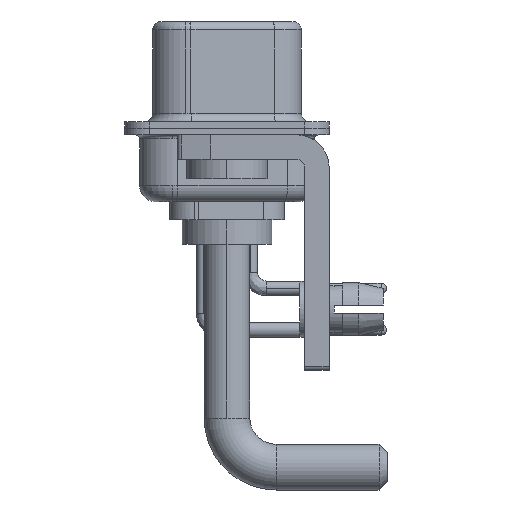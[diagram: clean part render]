
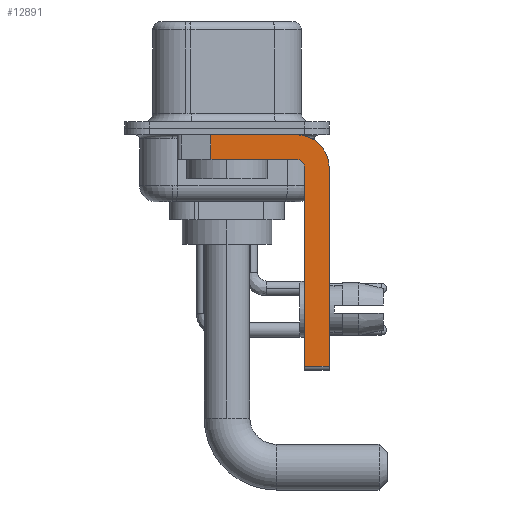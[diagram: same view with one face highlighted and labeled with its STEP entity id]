
A CAD part, left-side view. The second image highlights one B-rep face of the part: STEP entity #12891.
In plain terms, the highlighted planar face has unit normal (-1, 0, 0).
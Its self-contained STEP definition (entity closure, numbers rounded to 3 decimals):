
#320 = CARTESIAN_POINT ( 'NONE',  ( -2.9, -4.25, -2.4 ) ) ;
#941 = ORIENTED_EDGE ( 'NONE', *, *, #22098, .T. ) ;
#2034 = VECTOR ( 'NONE', #27669, 1000. ) ;
#2290 = CARTESIAN_POINT ( 'NONE',  ( -2.9, -4.25, -14.55 ) ) ;
#2913 = LINE ( 'NONE', #7847, #25503 ) ;
#4071 = CARTESIAN_POINT ( 'NONE',  ( -2.9, 0.978, -1.9 ) ) ;
#4389 = ORIENTED_EDGE ( 'NONE', *, *, #28642, .F. ) ;
#4575 = CARTESIAN_POINT ( 'NONE',  ( -2.9, -4.25, -2.4 ) ) ;
#4962 = PLANE ( 'NONE',  #6424 ) ;
#5772 = CARTESIAN_POINT ( 'NONE',  ( -2.9, -4.25, -1.9 ) ) ;
#6424 = AXIS2_PLACEMENT_3D ( 'NONE', #320, #7862, #24364 ) ;
#6675 = EDGE_CURVE ( 'NONE', #24162, #13296, #2913, .T. ) ;
#6744 = VECTOR ( 'NONE', #20681, 1000. ) ;
#7289 = VERTEX_POINT ( 'NONE', #16029 ) ;
#7725 = EDGE_CURVE ( 'NONE', #24919, #7289, #20651, .T. ) ;
#7847 = CARTESIAN_POINT ( 'NONE',  ( -2.9, 0.978, -1.9 ) ) ;
#7862 = DIRECTION ( 'NONE',  ( 1., 0., 0. ) ) ;
#8872 = CARTESIAN_POINT ( 'NONE',  ( -2.9, -4.25, -1.9 ) ) ;
#8944 = CARTESIAN_POINT ( 'NONE',  ( -2.9, -4.75, -14.8 ) ) ;
#10018 = EDGE_LOOP ( 'NONE', ( #18053, #20762, #11144, #4389, #27087, #941, #21379, #15560 ) ) ;
#11144 = ORIENTED_EDGE ( 'NONE', *, *, #27880, .F. ) ;
#11260 = CARTESIAN_POINT ( 'NONE',  ( -2.9, -6.25, -2.4 ) ) ;
#11601 = VECTOR ( 'NONE', #16126, 1000. ) ;
#12143 = EDGE_CURVE ( 'NONE', #24162, #20362, #23006, .T. ) ;
#12891 = ADVANCED_FACE ( 'NONE', ( #26078 ), #4962, .F. ) ;
#13296 = VERTEX_POINT ( 'NONE', #4071 ) ;
#13575 = LINE ( 'NONE', #11260, #6744 ) ;
#14870 = CIRCLE ( 'NONE', #25709, 2. ) ;
#15001 = EDGE_CURVE ( 'NONE', #20362, #17373, #14870, .T. ) ;
#15560 = ORIENTED_EDGE ( 'NONE', *, *, #15001, .F. ) ;
#15699 = DIRECTION ( 'NONE',  ( -1., 0., 0. ) ) ;
#15978 = LINE ( 'NONE', #2290, #11601 ) ;
#16029 = CARTESIAN_POINT ( 'NONE',  ( -2.9, -4.75, -2.4 ) ) ;
#16126 = DIRECTION ( 'NONE',  ( 0., -1., 0. ) ) ;
#17188 = CARTESIAN_POINT ( 'NONE',  ( -2.9, -4.75, -14.55 ) ) ;
#17373 = VERTEX_POINT ( 'NONE', #17679 ) ;
#17679 = CARTESIAN_POINT ( 'NONE',  ( -2.9, -6.25, -2.4 ) ) ;
#18053 = ORIENTED_EDGE ( 'NONE', *, *, #12143, .F. ) ;
#18065 = CIRCLE ( 'NONE', #19057, 0.5 ) ;
#18320 = DIRECTION ( 'NONE',  ( 0., 0., 1. ) ) ;
#19057 = AXIS2_PLACEMENT_3D ( 'NONE', #22949, #15699, #22507 ) ;
#20362 = VERTEX_POINT ( 'NONE', #22971 ) ;
#20651 = LINE ( 'NONE', #8944, #28042 ) ;
#20681 = DIRECTION ( 'NONE',  ( 0., 0., -1. ) ) ;
#20762 = ORIENTED_EDGE ( 'NONE', *, *, #6675, .T. ) ;
#21214 = DIRECTION ( 'NONE',  ( 0., 0., -1. ) ) ;
#21365 = DIRECTION ( 'NONE',  ( 1., 0., 0. ) ) ;
#21379 = ORIENTED_EDGE ( 'NONE', *, *, #28139, .F. ) ;
#22098 = EDGE_CURVE ( 'NONE', #24919, #25786, #15978, .T. ) ;
#22368 = VERTEX_POINT ( 'NONE', #8872 ) ;
#22507 = DIRECTION ( 'NONE',  ( 0., 0., 1. ) ) ;
#22949 = CARTESIAN_POINT ( 'NONE',  ( -2.9, -4.25, -2.4 ) ) ;
#22971 = CARTESIAN_POINT ( 'NONE',  ( -2.9, -4.25, -0.4 ) ) ;
#23006 = LINE ( 'NONE', #27955, #2034 ) ;
#23256 = CARTESIAN_POINT ( 'NONE',  ( -2.9, 0.978, -0.4 ) ) ;
#24162 = VERTEX_POINT ( 'NONE', #23256 ) ;
#24364 = DIRECTION ( 'NONE',  ( 0., 0., -1. ) ) ;
#24375 = CARTESIAN_POINT ( 'NONE',  ( -2.9, -6.25, -14.55 ) ) ;
#24919 = VERTEX_POINT ( 'NONE', #17188 ) ;
#25503 = VECTOR ( 'NONE', #28533, 1000. ) ;
#25709 = AXIS2_PLACEMENT_3D ( 'NONE', #4575, #21365, #21214 ) ;
#25786 = VERTEX_POINT ( 'NONE', #24375 ) ;
#26078 = FACE_OUTER_BOUND ( 'NONE', #10018, .T. ) ;
#26758 = DIRECTION ( 'NONE',  ( 0., 1., 0. ) ) ;
#26900 = LINE ( 'NONE', #5772, #28409 ) ;
#27087 = ORIENTED_EDGE ( 'NONE', *, *, #7725, .F. ) ;
#27669 = DIRECTION ( 'NONE',  ( 0., -1., 0. ) ) ;
#27880 = EDGE_CURVE ( 'NONE', #22368, #13296, #26900, .T. ) ;
#27955 = CARTESIAN_POINT ( 'NONE',  ( -2.9, 3., -0.4 ) ) ;
#28042 = VECTOR ( 'NONE', #18320, 1000. ) ;
#28139 = EDGE_CURVE ( 'NONE', #17373, #25786, #13575, .T. ) ;
#28409 = VECTOR ( 'NONE', #26758, 1000. ) ;
#28533 = DIRECTION ( 'NONE',  ( 0., 0., -1. ) ) ;
#28642 = EDGE_CURVE ( 'NONE', #7289, #22368, #18065, .T. ) ;
